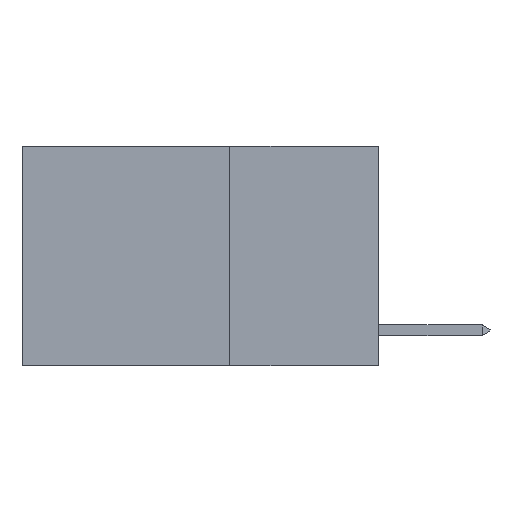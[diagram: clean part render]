
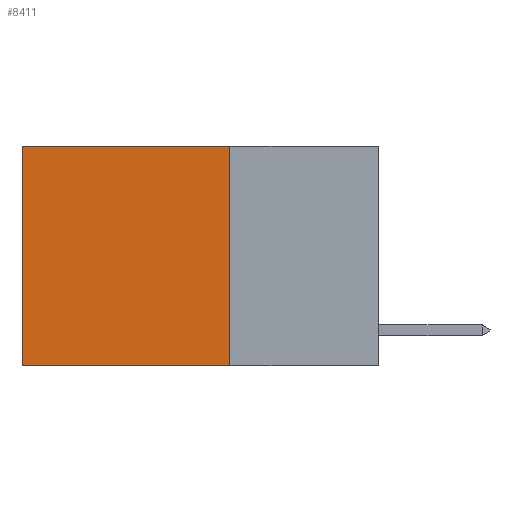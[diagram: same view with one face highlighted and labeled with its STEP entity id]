
A CAD part, left-side view. The second image highlights one B-rep face of the part: STEP entity #8411.
In plain terms, the highlighted planar face has unit normal (-1, 0, 0).
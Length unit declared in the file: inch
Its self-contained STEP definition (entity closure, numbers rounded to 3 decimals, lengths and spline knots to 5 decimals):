
#532 = LINE ( 'NONE', #14054, #6963 ) ;
#1185 = ORIENTED_EDGE ( 'NONE', *, *, #17535, .F. ) ;
#1654 = VECTOR ( 'NONE', #21054, 39.37008 ) ;
#1777 = VERTEX_POINT ( 'NONE', #17261 ) ;
#2879 = CARTESIAN_POINT ( 'NONE',  ( 0.2625, 0.6, -0.37 ) ) ;
#4229 = VECTOR ( 'NONE', #25656, 39.37008 ) ;
#5064 = CARTESIAN_POINT ( 'NONE',  ( 0.2625, 0.25, 0. ) ) ;
#5251 = LINE ( 'NONE', #21246, #4229 ) ;
#6275 = VERTEX_POINT ( 'NONE', #21280 ) ;
#6419 = EDGE_LOOP ( 'NONE', ( #16862, #1185, #18954, #20110 ) ) ;
#6717 = EDGE_CURVE ( 'NONE', #12294, #1777, #532, .T. ) ;
#6963 = VECTOR ( 'NONE', #21244, 39.37008 ) ;
#8411 = ADVANCED_FACE ( 'NONE', ( #9898 ), #16385, .F. ) ;
#9898 = FACE_OUTER_BOUND ( 'NONE', #6419, .T. ) ;
#12294 = VERTEX_POINT ( 'NONE', #27912 ) ;
#12799 = VERTEX_POINT ( 'NONE', #2879 ) ;
#12866 = VECTOR ( 'NONE', #25999, 39.37008 ) ;
#14054 = CARTESIAN_POINT ( 'NONE',  ( 0.2625, 0.25, 0. ) ) ;
#14529 = CARTESIAN_POINT ( 'NONE',  ( 0.2625, 0.25, 0. ) ) ;
#16385 = PLANE ( 'NONE',  #23942 ) ;
#16532 = DIRECTION ( 'NONE',  ( 0., 0., -1. ) ) ;
#16649 = EDGE_CURVE ( 'NONE', #12294, #6275, #17178, .T. ) ;
#16862 = ORIENTED_EDGE ( 'NONE', *, *, #24046, .T. ) ;
#17178 = LINE ( 'NONE', #14529, #12866 ) ;
#17261 = CARTESIAN_POINT ( 'NONE',  ( 0.2625, 0.25, -0.37 ) ) ;
#17535 = EDGE_CURVE ( 'NONE', #1777, #12799, #19147, .T. ) ;
#18708 = CARTESIAN_POINT ( 'NONE',  ( 0.2625, 0.25, -0.37 ) ) ;
#18954 = ORIENTED_EDGE ( 'NONE', *, *, #6717, .F. ) ;
#19147 = LINE ( 'NONE', #18708, #1654 ) ;
#20110 = ORIENTED_EDGE ( 'NONE', *, *, #16649, .T. ) ;
#21054 = DIRECTION ( 'NONE',  ( 0., 1., 0. ) ) ;
#21244 = DIRECTION ( 'NONE',  ( 0., 0., -1. ) ) ;
#21246 = CARTESIAN_POINT ( 'NONE',  ( 0.2625, 0.6, 0. ) ) ;
#21280 = CARTESIAN_POINT ( 'NONE',  ( 0.2625, 0.6, 0. ) ) ;
#23942 = AXIS2_PLACEMENT_3D ( 'NONE', #5064, #27842, #16532 ) ;
#24046 = EDGE_CURVE ( 'NONE', #6275, #12799, #5251, .T. ) ;
#25656 = DIRECTION ( 'NONE',  ( 0., 0., -1. ) ) ;
#25999 = DIRECTION ( 'NONE',  ( 0., 1., 0. ) ) ;
#27842 = DIRECTION ( 'NONE',  ( 1., 0., 0. ) ) ;
#27912 = CARTESIAN_POINT ( 'NONE',  ( 0.2625, 0.25, 0. ) ) ;
